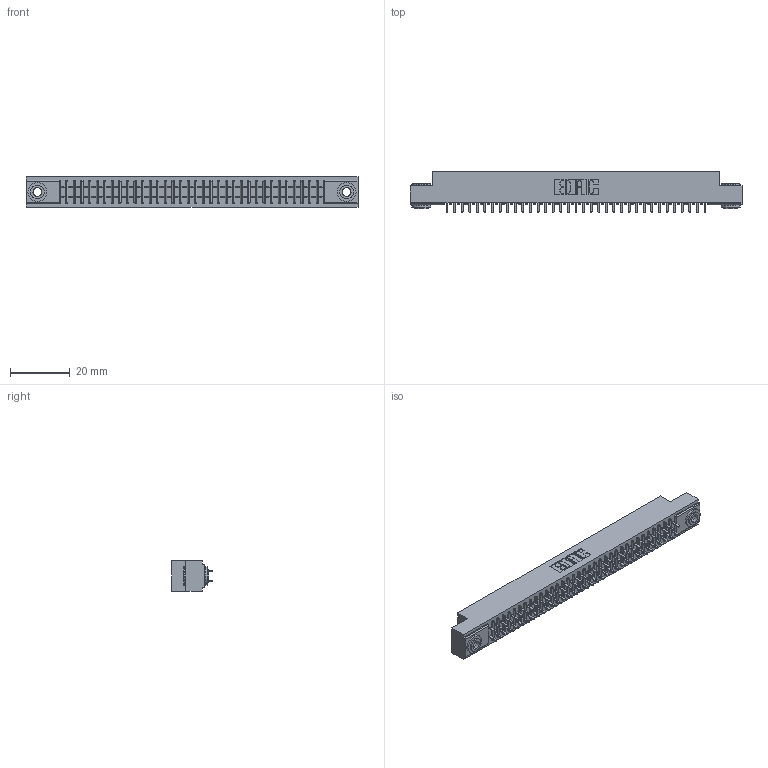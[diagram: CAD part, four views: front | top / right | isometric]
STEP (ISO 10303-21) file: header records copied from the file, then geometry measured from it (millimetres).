
FILE_DESCRIPTION (( 'STEP AP203' ), '1' );
FILE_NAME ('341-070-524-203.STEP', '2018-08-07T19:33:38', ( '' ), ( '' ), 'SwSTEP 2.0', 'SolidWorks 2016', '' );
FILE_SCHEMA (( 'CONFIG_CONTROL_DESIGN' ));
Length unit declared in the file: inch
Products named in the file (4): 341 Part_.156 (3.96) Dia Mounting Holes; 341-292-001_341-292-124; 345-250-002_345-250-002-102; 341-070-524-203
Assembly tree (73 placements, depth 2):
  341-070-524-203
    341 Part_.156 (3.96) Dia Mounting Holes
    341-292-001_341-292-124  x70
    345-250-002_345-250-002-102  x2
Bounding box: 111.12 x 13.64 x 10.16 mm (x, y, z)
Volume: 8194.5 mm3; surface area: 14434.7 mm2
Topology: 73 solids, 73 shells, 4788 faces, 13833 edges, 8958 vertices
Faces by surface type: plane 2892, cylinder 1748, sphere 72, torus 68, cone 8
Entity records: 44355 total; most frequent: CARTESIAN_POINT 7354, ORIENTED_EDGE 7298, DIRECTION 7157, EDGE_CURVE 3649, VECTOR 2931, LINE 2931, VERTEX_POINT 2310, AXIS2_PLACEMENT_3D 2113
